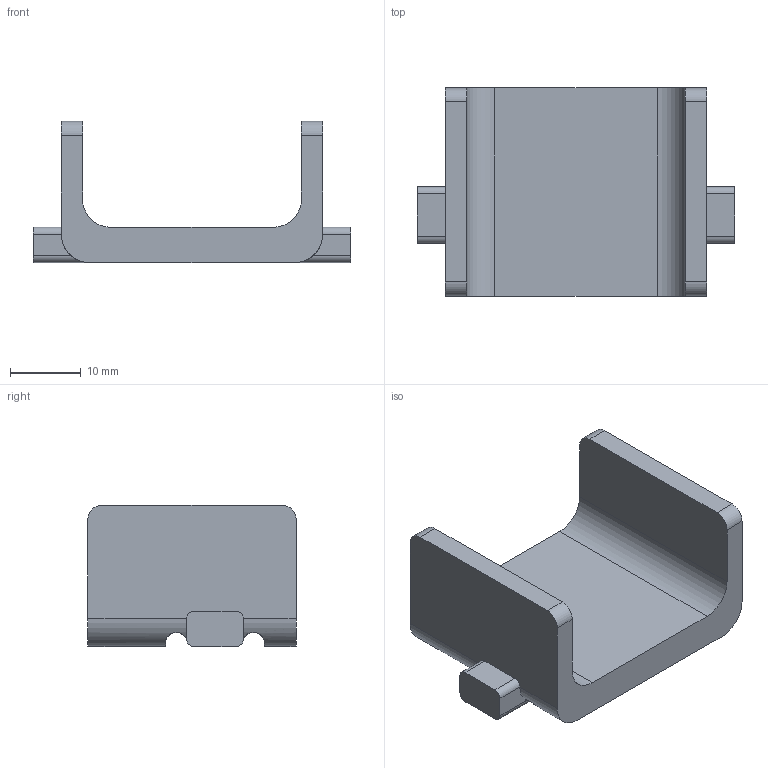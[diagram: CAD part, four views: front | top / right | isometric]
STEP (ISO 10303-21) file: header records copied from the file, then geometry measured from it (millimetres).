
FILE_DESCRIPTION((''),'2;1');
FILE_NAME('PM422BarrelCatch2.stp','2015-08-22T19:06:15',('JamesRPatrick'),(''),'Autodesk Inventor 2012','Autodesk Inventor 2012','');
FILE_SCHEMA(('AUTOMOTIVE_DESIGN { 1 0 10303 214 1 1 1 1 }'));
Length unit declared in the file: millimetre
Products named in the file (1): PM422BarrelCatch2
Bounding box: 45 x 29.5 x 20 mm (x, y, z)
Volume: 8111.6 mm3; surface area: 4958.2 mm2
Topology: 1 solids, 1 shells, 44 faces, 122 edges, 80 vertices
Faces by surface type: plane 24, cylinder 20
Entity records: 1528 total; most frequent: CARTESIAN_POINT 363, ORIENTED_EDGE 244, DIRECTION 236, EDGE_CURVE 122, AXIS2_PLACEMENT_3D 81, VERTEX_POINT 80, VECTOR 74, LINE 74
